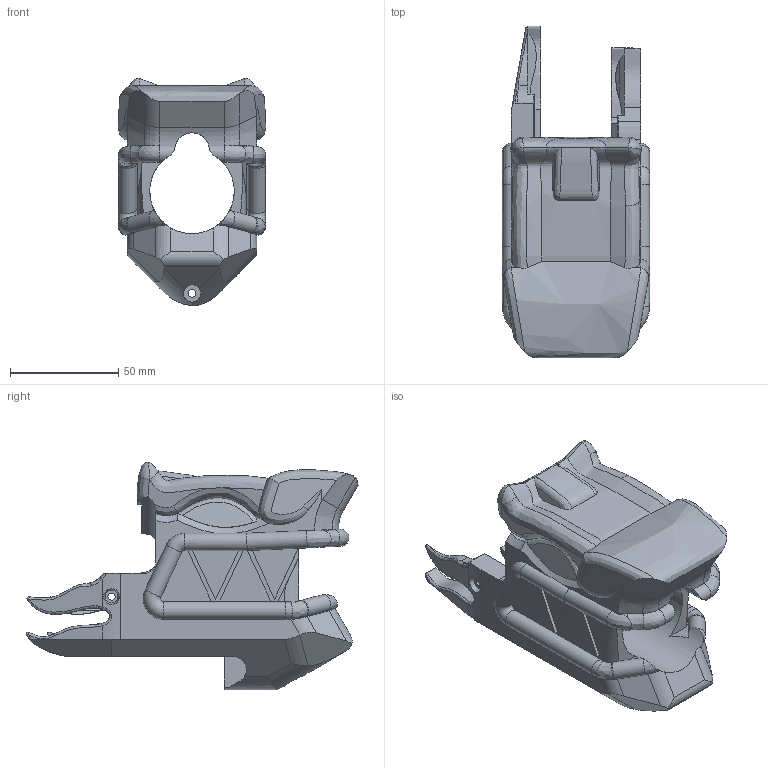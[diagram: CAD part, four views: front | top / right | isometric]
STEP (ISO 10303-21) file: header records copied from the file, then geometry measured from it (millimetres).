
FILE_DESCRIPTION(/* description */ (''),/* implementation_level */ '2;1');
FILE_NAME(/* name */ 'KG99mini-Tec9mini-AB10-MulanDragon.step',/* time_stamp */ '2025-05-18T02:20:14-04:00',/* author */ (''),/* organization */ (''),/* preprocessor_version */ 'ST-DEVELOPER v20.1',/* originating_system */ 'Autodesk Translation Framework v14.4.0.0',/* authorisation */ '');
FILE_SCHEMA (('AUTOMOTIVE_DESIGN { 1 0 10303 214 3 1 1 }'));
Length unit declared in the file: millimetre
Products named in the file (1): Dragon6Mini1
Bounding box: 68.2 x 153.41 x 105.05 mm (x, y, z)
Volume: 303587.9 mm3; surface area: 59062.1 mm2
Topology: 1 solids, 1 shells, 295 faces, 931 edges, 633 vertices
Faces by surface type: plane 132, bspline 100, cylinder 53, torus 6, cone 4
Full cylindrical faces by diameter (mm): 3.3 x2, 3.5 x1, 8 x1
Entity records: 30204 total; most frequent: CARTESIAN_POINT 22708, ORIENTED_EDGE 1850, DIRECTION 1162, EDGE_CURVE 925, VERTEX_POINT 633, AXIS2_PLACEMENT_3D 403, B_SPLINE_CURVE_WITH_KNOTS 362, LINE 356
